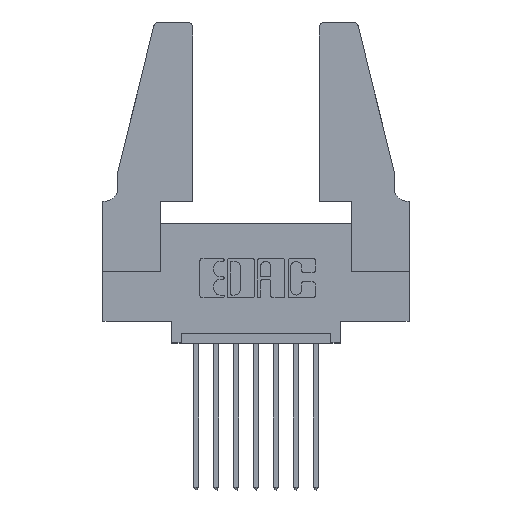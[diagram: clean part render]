
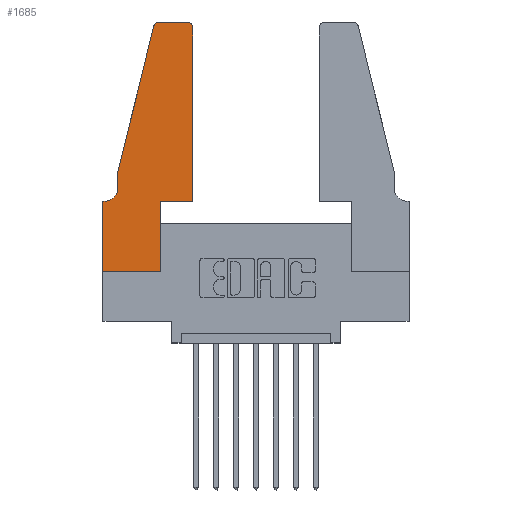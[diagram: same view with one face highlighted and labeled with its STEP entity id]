
A CAD part, top view. The second image highlights one B-rep face of the part: STEP entity #1685.
In plain terms, the highlighted planar face has unit normal (0, 0, 1).
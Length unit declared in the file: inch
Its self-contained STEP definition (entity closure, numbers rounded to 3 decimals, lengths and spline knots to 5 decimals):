
#85 = DIRECTION ( 'NONE',  ( -1., 0., 0. ) ) ;
#136 = DIRECTION ( 'NONE',  ( 0., 0., -1. ) ) ;
#324 = LINE ( 'NONE', #4328, #12022 ) ;
#334 = VECTOR ( 'NONE', #6678, 39.37008 ) ;
#611 = EDGE_CURVE ( 'NONE', #2546, #7133, #9833, .T. ) ;
#631 = DIRECTION ( 'NONE',  ( 0., -1., 0. ) ) ;
#707 = DIRECTION ( 'NONE',  ( 0., 0., 1. ) ) ;
#731 = CIRCLE ( 'NONE', #10933, 0.03 ) ;
#786 = VECTOR ( 'NONE', #1000, 39.37008 ) ;
#842 = ORIENTED_EDGE ( 'NONE', *, *, #5977, .T. ) ;
#1000 = DIRECTION ( 'NONE',  ( 0., 1., 0. ) ) ;
#1242 = EDGE_CURVE ( 'NONE', #8793, #3814, #3428, .T. ) ;
#1349 = CARTESIAN_POINT ( 'NONE',  ( 0.2865, 0.35, 0.37 ) ) ;
#1482 = VECTOR ( 'NONE', #9453, 39.37008 ) ;
#1523 = CARTESIAN_POINT ( 'NONE',  ( 0., 0., 0.37 ) ) ;
#1685 = ADVANCED_FACE ( 'NONE', ( #12161 ), #10468, .T. ) ;
#1833 = CARTESIAN_POINT ( 'NONE',  ( 0.284, 1.25, 0.37 ) ) ;
#2066 = LINE ( 'NONE', #10365, #10498 ) ;
#2112 = CARTESIAN_POINT ( 'NONE',  ( 0.4505, 0.35, 0.37 ) ) ;
#2124 = CARTESIAN_POINT ( 'NONE',  ( 0.0055, 0.35, 0.37 ) ) ;
#2128 = EDGE_CURVE ( 'NONE', #7167, #3486, #2066, .T. ) ;
#2205 = VERTEX_POINT ( 'NONE', #11530 ) ;
#2271 = LINE ( 'NONE', #7965, #4205 ) ;
#2311 = CARTESIAN_POINT ( 'NONE',  ( 0.4205, 1.22, 0.37 ) ) ;
#2546 = VERTEX_POINT ( 'NONE', #4204 ) ;
#2602 = ORIENTED_EDGE ( 'NONE', *, *, #8767, .T. ) ;
#2649 = DIRECTION ( 'NONE',  ( 1., 0., 0. ) ) ;
#2831 = EDGE_CURVE ( 'NONE', #4227, #2546, #8126, .T. ) ;
#2866 = LINE ( 'NONE', #7761, #334 ) ;
#2871 = DIRECTION ( 'NONE',  ( 1., 0., 0. ) ) ;
#3006 = CARTESIAN_POINT ( 'NONE',  ( 0.0055, 0.42, 0.37 ) ) ;
#3173 = VERTEX_POINT ( 'NONE', #2112 ) ;
#3317 = EDGE_LOOP ( 'NONE', ( #7177, #842, #9379, #2602, #10261, #8345, #4326, #6612, #6185, #8712, #7160, #3488 ) ) ;
#3374 = AXIS2_PLACEMENT_3D ( 'NONE', #2311, #8951, #8148 ) ;
#3428 = LINE ( 'NONE', #8764, #7129 ) ;
#3486 = VERTEX_POINT ( 'NONE', #3540 ) ;
#3488 = ORIENTED_EDGE ( 'NONE', *, *, #2831, .T. ) ;
#3540 = CARTESIAN_POINT ( 'NONE',  ( 0., 0.35, 0.37 ) ) ;
#3628 = EDGE_CURVE ( 'NONE', #6268, #9871, #5004, .T. ) ;
#3814 = VERTEX_POINT ( 'NONE', #7524 ) ;
#4118 = DIRECTION ( 'NONE',  ( -1., 0., 0. ) ) ;
#4204 = CARTESIAN_POINT ( 'NONE',  ( 0.4205, 1.25, 0.37 ) ) ;
#4205 = VECTOR ( 'NONE', #4208, 39.37008 ) ;
#4208 = DIRECTION ( 'NONE',  ( 0., -1., 0. ) ) ;
#4227 = VERTEX_POINT ( 'NONE', #5668 ) ;
#4326 = ORIENTED_EDGE ( 'NONE', *, *, #11486, .T. ) ;
#4328 = CARTESIAN_POINT ( 'NONE',  ( 0., 0., 0.37 ) ) ;
#4630 = CARTESIAN_POINT ( 'NONE',  ( 0.0755, 0.5, 0.37 ) ) ;
#5004 = LINE ( 'NONE', #7588, #9298 ) ;
#5655 = LINE ( 'NONE', #9534, #786 ) ;
#5668 = CARTESIAN_POINT ( 'NONE',  ( 0.4505, 1.22, 0.37 ) ) ;
#5759 = EDGE_CURVE ( 'NONE', #3814, #8889, #6644, .T. ) ;
#5855 = CIRCLE ( 'NONE', #7510, 0.07 ) ;
#5977 = EDGE_CURVE ( 'NONE', #7133, #6268, #731, .T. ) ;
#6051 = DIRECTION ( 'NONE',  ( 1., 0., 0. ) ) ;
#6185 = ORIENTED_EDGE ( 'NONE', *, *, #5759, .T. ) ;
#6268 = VERTEX_POINT ( 'NONE', #11420 ) ;
#6396 = VECTOR ( 'NONE', #4118, 39.37008 ) ;
#6608 = AXIS2_PLACEMENT_3D ( 'NONE', #9615, #7577, #2871 ) ;
#6612 = ORIENTED_EDGE ( 'NONE', *, *, #1242, .T. ) ;
#6644 = LINE ( 'NONE', #8499, #1482 ) ;
#6678 = DIRECTION ( 'NONE',  ( 1., 0., 0. ) ) ;
#7129 = VECTOR ( 'NONE', #6051, 39.37008 ) ;
#7133 = VERTEX_POINT ( 'NONE', #1833 ) ;
#7134 = EDGE_CURVE ( 'NONE', #2205, #7167, #5855, .T. ) ;
#7160 = ORIENTED_EDGE ( 'NONE', *, *, #9078, .T. ) ;
#7167 = VERTEX_POINT ( 'NONE', #2124 ) ;
#7177 = ORIENTED_EDGE ( 'NONE', *, *, #611, .T. ) ;
#7510 = AXIS2_PLACEMENT_3D ( 'NONE', #3006, #136, #85 ) ;
#7524 = CARTESIAN_POINT ( 'NONE',  ( 0.2865, 0., 0.37 ) ) ;
#7577 = DIRECTION ( 'NONE',  ( 0., 0., 1. ) ) ;
#7588 = CARTESIAN_POINT ( 'NONE',  ( 0.0755, 0.5, 0.37 ) ) ;
#7761 = CARTESIAN_POINT ( 'NONE',  ( 0.4505, 0.35, 0.37 ) ) ;
#7965 = CARTESIAN_POINT ( 'NONE',  ( 0.0755, 0.5, 0.37 ) ) ;
#8126 = CIRCLE ( 'NONE', #3374, 0.03 ) ;
#8148 = DIRECTION ( 'NONE',  ( 1., 0., 0. ) ) ;
#8345 = ORIENTED_EDGE ( 'NONE', *, *, #2128, .T. ) ;
#8499 = CARTESIAN_POINT ( 'NONE',  ( 0.2865, 0.35, 0.37 ) ) ;
#8547 = DIRECTION ( 'NONE',  ( -0.239, -0.971, 0. ) ) ;
#8566 = DIRECTION ( 'NONE',  ( -1., 0., 0. ) ) ;
#8712 = ORIENTED_EDGE ( 'NONE', *, *, #9307, .T. ) ;
#8764 = CARTESIAN_POINT ( 'NONE',  ( 0., 0., 0.37 ) ) ;
#8767 = EDGE_CURVE ( 'NONE', #9871, #2205, #2271, .T. ) ;
#8793 = VERTEX_POINT ( 'NONE', #1523 ) ;
#8889 = VERTEX_POINT ( 'NONE', #1349 ) ;
#8951 = DIRECTION ( 'NONE',  ( 0., 0., 1. ) ) ;
#9078 = EDGE_CURVE ( 'NONE', #3173, #4227, #5655, .T. ) ;
#9298 = VECTOR ( 'NONE', #8547, 39.37008 ) ;
#9307 = EDGE_CURVE ( 'NONE', #8889, #3173, #2866, .T. ) ;
#9379 = ORIENTED_EDGE ( 'NONE', *, *, #3628, .T. ) ;
#9453 = DIRECTION ( 'NONE',  ( 0., 1., 0. ) ) ;
#9534 = CARTESIAN_POINT ( 'NONE',  ( 0.4505, 0.35, 0.37 ) ) ;
#9615 = CARTESIAN_POINT ( 'NONE',  ( 0., 0.35, 0.37 ) ) ;
#9833 = LINE ( 'NONE', #10811, #6396 ) ;
#9871 = VERTEX_POINT ( 'NONE', #4630 ) ;
#10261 = ORIENTED_EDGE ( 'NONE', *, *, #7134, .T. ) ;
#10365 = CARTESIAN_POINT ( 'NONE',  ( 0.0755, 0.35, 0.37 ) ) ;
#10468 = PLANE ( 'NONE',  #6608 ) ;
#10498 = VECTOR ( 'NONE', #8566, 39.37008 ) ;
#10811 = CARTESIAN_POINT ( 'NONE',  ( 0.2605, 1.25, 0.37 ) ) ;
#10933 = AXIS2_PLACEMENT_3D ( 'NONE', #11050, #707, #2649 ) ;
#11050 = CARTESIAN_POINT ( 'NONE',  ( 0.284, 1.22, 0.37 ) ) ;
#11420 = CARTESIAN_POINT ( 'NONE',  ( 0.25487, 1.22718, 0.37 ) ) ;
#11486 = EDGE_CURVE ( 'NONE', #3486, #8793, #324, .T. ) ;
#11530 = CARTESIAN_POINT ( 'NONE',  ( 0.0755, 0.42, 0.37 ) ) ;
#12022 = VECTOR ( 'NONE', #631, 39.37008 ) ;
#12161 = FACE_OUTER_BOUND ( 'NONE', #3317, .T. ) ;
